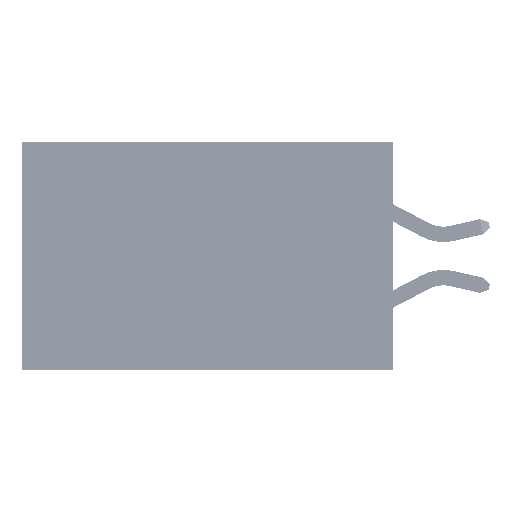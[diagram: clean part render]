
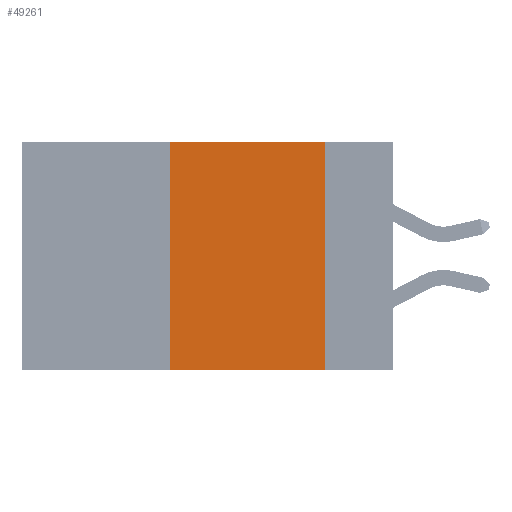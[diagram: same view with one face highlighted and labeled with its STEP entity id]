
A CAD part, left-side view. The second image highlights one B-rep face of the part: STEP entity #49261.
In plain terms, the highlighted planar face has unit normal (-1, 0, 0).
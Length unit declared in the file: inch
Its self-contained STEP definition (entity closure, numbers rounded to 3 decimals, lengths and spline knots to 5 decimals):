
#166 = EDGE_CURVE ( 'NONE', #13081, #39013, #41079, .T. ) ;
#1295 = DIRECTION ( 'NONE',  ( 0., 0., -1. ) ) ;
#1397 = EDGE_LOOP ( 'NONE', ( #11481, #4426, #29432, #45916 ) ) ;
#1427 = DIRECTION ( 'NONE',  ( 0., -1., 0. ) ) ;
#2727 = DIRECTION ( 'NONE',  ( 1., 0., 0. ) ) ;
#4426 = ORIENTED_EDGE ( 'NONE', *, *, #45355, .F. ) ;
#5456 = CARTESIAN_POINT ( 'NONE',  ( 0., 0.11, 0. ) ) ;
#5988 = VERTEX_POINT ( 'NONE', #14282 ) ;
#6264 = CARTESIAN_POINT ( 'NONE',  ( 0., 0.6, 0. ) ) ;
#7578 = EDGE_CURVE ( 'NONE', #28372, #5988, #9958, .T. ) ;
#9958 = LINE ( 'NONE', #20150, #42358 ) ;
#11481 = ORIENTED_EDGE ( 'NONE', *, *, #7578, .F. ) ;
#12507 = DIRECTION ( 'NONE',  ( 0., -1., 0. ) ) ;
#13081 = VERTEX_POINT ( 'NONE', #37815 ) ;
#13388 = DIRECTION ( 'NONE',  ( 0., 0., 1. ) ) ;
#14282 = CARTESIAN_POINT ( 'NONE',  ( 0., 0.11, -0.37 ) ) ;
#16884 = CARTESIAN_POINT ( 'NONE',  ( 0., 0.36, 0. ) ) ;
#19996 = VECTOR ( 'NONE', #13388, 39.37008 ) ;
#20120 = CARTESIAN_POINT ( 'NONE',  ( 0., 0.6, -0.37 ) ) ;
#20126 = EDGE_CURVE ( 'NONE', #13081, #5988, #41149, .T. ) ;
#20150 = CARTESIAN_POINT ( 'NONE',  ( 0., 0.11, 0. ) ) ;
#22055 = FACE_OUTER_BOUND ( 'NONE', #1397, .T. ) ;
#28372 = VERTEX_POINT ( 'NONE', #5456 ) ;
#29432 = ORIENTED_EDGE ( 'NONE', *, *, #166, .F. ) ;
#31611 = CARTESIAN_POINT ( 'NONE',  ( 0., 0.6, 0. ) ) ;
#33367 = VECTOR ( 'NONE', #1427, 39.37008 ) ;
#34595 = VECTOR ( 'NONE', #12507, 39.37008 ) ;
#37232 = DIRECTION ( 'NONE',  ( 0., 0., -1. ) ) ;
#37815 = CARTESIAN_POINT ( 'NONE',  ( 0., 0.36, -0.37 ) ) ;
#39013 = VERTEX_POINT ( 'NONE', #39453 ) ;
#39453 = CARTESIAN_POINT ( 'NONE',  ( 0., 0.36, 0. ) ) ;
#40454 = PLANE ( 'NONE',  #43480 ) ;
#41079 = LINE ( 'NONE', #16884, #19996 ) ;
#41149 = LINE ( 'NONE', #20120, #33367 ) ;
#42358 = VECTOR ( 'NONE', #1295, 39.37008 ) ;
#43480 = AXIS2_PLACEMENT_3D ( 'NONE', #6264, #2727, #37232 ) ;
#45355 = EDGE_CURVE ( 'NONE', #39013, #28372, #45989, .T. ) ;
#45916 = ORIENTED_EDGE ( 'NONE', *, *, #20126, .T. ) ;
#45989 = LINE ( 'NONE', #31611, #34595 ) ;
#49261 = ADVANCED_FACE ( 'NONE', ( #22055 ), #40454, .F. ) ;
